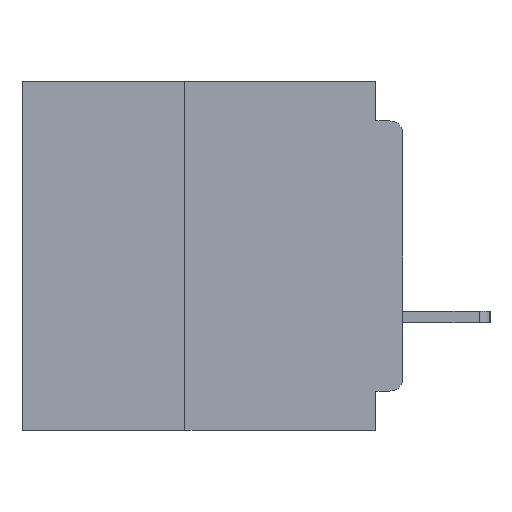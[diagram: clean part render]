
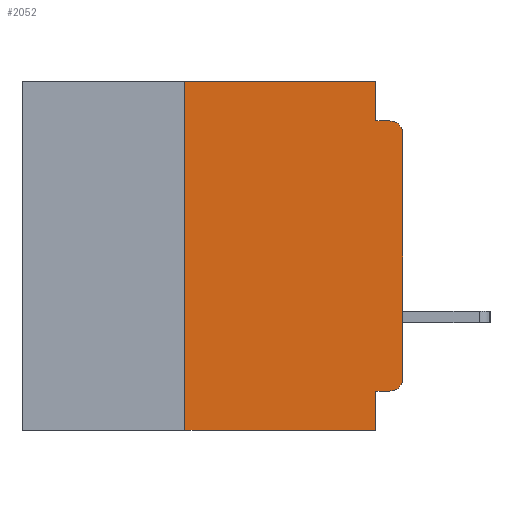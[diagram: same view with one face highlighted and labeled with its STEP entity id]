
A CAD part, left-side view. The second image highlights one B-rep face of the part: STEP entity #2052.
In plain terms, the highlighted planar face has unit normal (-1, 0, 0).
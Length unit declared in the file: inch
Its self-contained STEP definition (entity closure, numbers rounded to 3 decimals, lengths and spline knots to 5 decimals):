
#41 = VECTOR ( 'NONE', #17852, 39.37008 ) ;
#718 = CARTESIAN_POINT ( 'NONE',  ( 0., 0.437, 0. ) ) ;
#741 = VECTOR ( 'NONE', #25743, 39.37008 ) ;
#821 = VECTOR ( 'NONE', #36964, 39.37008 ) ;
#1091 = EDGE_CURVE ( 'NONE', #22516, #11546, #31921, .T. ) ;
#1758 = DIRECTION ( 'NONE',  ( 0., -1., 0. ) ) ;
#2052 = ADVANCED_FACE ( 'NONE', ( #36712 ), #19322, .F. ) ;
#2142 = CARTESIAN_POINT ( 'NONE',  ( 0., 0., -0.34 ) ) ;
#2536 = VERTEX_POINT ( 'NONE', #6283 ) ;
#2996 = CARTESIAN_POINT ( 'NONE',  ( 0., 0.015, -0.06 ) ) ;
#3086 = CARTESIAN_POINT ( 'NONE',  ( 0., 0.25, -0.4 ) ) ;
#3292 = VECTOR ( 'NONE', #17595, 39.37008 ) ;
#3481 = EDGE_LOOP ( 'NONE', ( #5738, #8328, #18645, #39398, #22330, #10703, #18398, #12376, #6580, #5836 ) ) ;
#4345 = CARTESIAN_POINT ( 'NONE',  ( 0., 0.25, 0. ) ) ;
#4691 = VECTOR ( 'NONE', #22157, 39.37008 ) ;
#4881 = VECTOR ( 'NONE', #1758, 39.37008 ) ;
#5738 = ORIENTED_EDGE ( 'NONE', *, *, #38581, .T. ) ;
#5829 = LINE ( 'NONE', #38864, #4881 ) ;
#5836 = ORIENTED_EDGE ( 'NONE', *, *, #35112, .T. ) ;
#6084 = VERTEX_POINT ( 'NONE', #33279 ) ;
#6117 = DIRECTION ( 'NONE',  ( 0., 0., -1. ) ) ;
#6283 = CARTESIAN_POINT ( 'NONE',  ( 0., 0.031, 0. ) ) ;
#6580 = ORIENTED_EDGE ( 'NONE', *, *, #1091, .F. ) ;
#7508 = DIRECTION ( 'NONE',  ( 0., -1., 0. ) ) ;
#7591 = VERTEX_POINT ( 'NONE', #4345 ) ;
#7886 = CIRCLE ( 'NONE', #32364, 0.015 ) ;
#8328 = ORIENTED_EDGE ( 'NONE', *, *, #10858, .T. ) ;
#8399 = CARTESIAN_POINT ( 'NONE',  ( 0., 0., 0. ) ) ;
#8608 = EDGE_CURVE ( 'NONE', #2536, #30881, #12922, .T. ) ;
#8696 = EDGE_CURVE ( 'NONE', #11546, #6084, #25605, .T. ) ;
#10107 = DIRECTION ( 'NONE',  ( 1., 0., 0. ) ) ;
#10212 = CARTESIAN_POINT ( 'NONE',  ( 0., 0.031, -0.4 ) ) ;
#10703 = ORIENTED_EDGE ( 'NONE', *, *, #35642, .F. ) ;
#10858 = EDGE_CURVE ( 'NONE', #34703, #17474, #7886, .T. ) ;
#11546 = VERTEX_POINT ( 'NONE', #34226 ) ;
#12376 = ORIENTED_EDGE ( 'NONE', *, *, #8696, .F. ) ;
#12789 = CARTESIAN_POINT ( 'NONE',  ( 0., 0.031, 0. ) ) ;
#12922 = LINE ( 'NONE', #12789, #4691 ) ;
#15863 = CARTESIAN_POINT ( 'NONE',  ( 0., 0.015, -0.34 ) ) ;
#16679 = CARTESIAN_POINT ( 'NONE',  ( 0., 0.437, 0. ) ) ;
#17341 = LINE ( 'NONE', #33869, #821 ) ;
#17474 = VERTEX_POINT ( 'NONE', #31196 ) ;
#17545 = AXIS2_PLACEMENT_3D ( 'NONE', #718, #10107, #31803 ) ;
#17595 = DIRECTION ( 'NONE',  ( 0., 0., 1. ) ) ;
#17852 = DIRECTION ( 'NONE',  ( 0., -1., 0. ) ) ;
#18398 = ORIENTED_EDGE ( 'NONE', *, *, #33635, .T. ) ;
#18645 = ORIENTED_EDGE ( 'NONE', *, *, #32541, .F. ) ;
#18999 = DIRECTION ( 'NONE',  ( 0., 0., -1. ) ) ;
#19322 = PLANE ( 'NONE',  #17545 ) ;
#19772 = LINE ( 'NONE', #8399, #3292 ) ;
#22157 = DIRECTION ( 'NONE',  ( 0., 0., -1. ) ) ;
#22330 = ORIENTED_EDGE ( 'NONE', *, *, #39673, .F. ) ;
#22516 = VERTEX_POINT ( 'NONE', #27904 ) ;
#22721 = VECTOR ( 'NONE', #38866, 39.37008 ) ;
#24740 = DIRECTION ( 'NONE',  ( -1., 0., 0. ) ) ;
#25571 = VECTOR ( 'NONE', #7508, 39.37008 ) ;
#25605 = LINE ( 'NONE', #10212, #741 ) ;
#25743 = DIRECTION ( 'NONE',  ( 0., 0., -1. ) ) ;
#26534 = CARTESIAN_POINT ( 'NONE',  ( 0., 0., -0.355 ) ) ;
#26568 = LINE ( 'NONE', #16679, #25571 ) ;
#27407 = CARTESIAN_POINT ( 'NONE',  ( 0., 0., -0.045 ) ) ;
#27850 = VERTEX_POINT ( 'NONE', #2142 ) ;
#27904 = CARTESIAN_POINT ( 'NONE',  ( 0., 0.015, -0.355 ) ) ;
#28047 = VERTEX_POINT ( 'NONE', #3086 ) ;
#28627 = CIRCLE ( 'NONE', #39465, 0.015 ) ;
#30881 = VERTEX_POINT ( 'NONE', #34636 ) ;
#31196 = CARTESIAN_POINT ( 'NONE',  ( 0., 0.015, -0.045 ) ) ;
#31803 = DIRECTION ( 'NONE',  ( 0., 0., -1. ) ) ;
#31921 = LINE ( 'NONE', #26534, #22721 ) ;
#32364 = AXIS2_PLACEMENT_3D ( 'NONE', #2996, #24740, #6117 ) ;
#32541 = EDGE_CURVE ( 'NONE', #30881, #17474, #39347, .T. ) ;
#33279 = CARTESIAN_POINT ( 'NONE',  ( 0., 0.031, -0.4 ) ) ;
#33635 = EDGE_CURVE ( 'NONE', #28047, #6084, #5829, .T. ) ;
#33869 = CARTESIAN_POINT ( 'NONE',  ( 0., 0.25, -0.4 ) ) ;
#34226 = CARTESIAN_POINT ( 'NONE',  ( 0., 0.031, -0.355 ) ) ;
#34636 = CARTESIAN_POINT ( 'NONE',  ( 0., 0.031, -0.045 ) ) ;
#34703 = VERTEX_POINT ( 'NONE', #38793 ) ;
#35112 = EDGE_CURVE ( 'NONE', #22516, #27850, #28627, .T. ) ;
#35642 = EDGE_CURVE ( 'NONE', #28047, #7591, #17341, .T. ) ;
#36712 = FACE_OUTER_BOUND ( 'NONE', #3481, .T. ) ;
#36964 = DIRECTION ( 'NONE',  ( 0., 0., 1. ) ) ;
#37545 = DIRECTION ( 'NONE',  ( -1., 0., 0. ) ) ;
#38581 = EDGE_CURVE ( 'NONE', #27850, #34703, #19772, .T. ) ;
#38793 = CARTESIAN_POINT ( 'NONE',  ( 0., 0., -0.06 ) ) ;
#38864 = CARTESIAN_POINT ( 'NONE',  ( 0., 0.437, -0.4 ) ) ;
#38866 = DIRECTION ( 'NONE',  ( 0., 1., 0. ) ) ;
#39347 = LINE ( 'NONE', #27407, #41 ) ;
#39398 = ORIENTED_EDGE ( 'NONE', *, *, #8608, .F. ) ;
#39465 = AXIS2_PLACEMENT_3D ( 'NONE', #15863, #37545, #18999 ) ;
#39673 = EDGE_CURVE ( 'NONE', #7591, #2536, #26568, .T. ) ;
